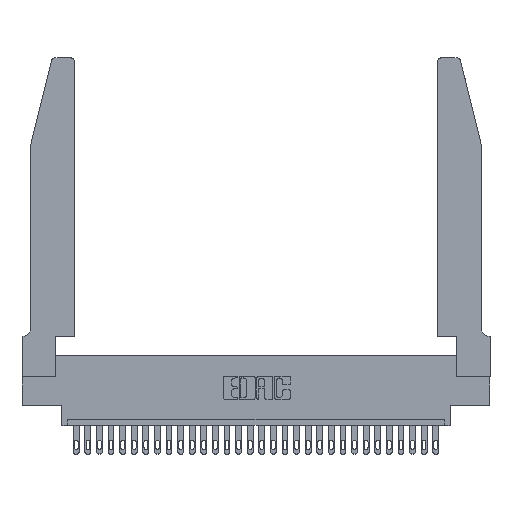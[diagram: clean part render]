
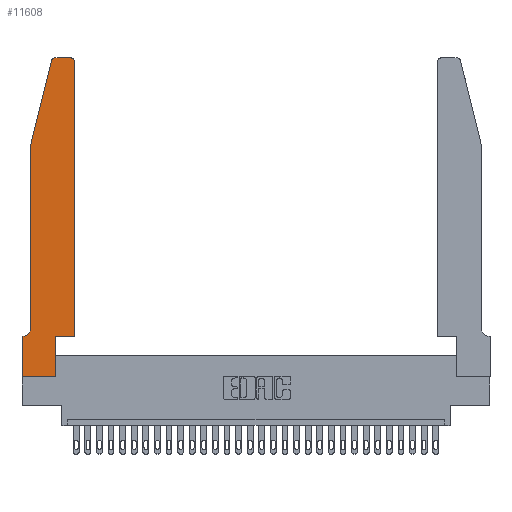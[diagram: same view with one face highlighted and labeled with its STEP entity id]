
A CAD part, top view. The second image highlights one B-rep face of the part: STEP entity #11608.
In plain terms, the highlighted planar face has unit normal (0, 0, 1).
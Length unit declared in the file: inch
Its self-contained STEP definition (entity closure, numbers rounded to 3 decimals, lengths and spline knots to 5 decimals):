
#44 = DIRECTION ( 'NONE',  ( 0., 0., 1. ) ) ;
#209 = EDGE_CURVE ( 'NONE', #25080, #17520, #10941, .T. ) ;
#1206 = VECTOR ( 'NONE', #19951, 39.37008 ) ;
#1261 = DIRECTION ( 'NONE',  ( -0.239, -0.971, 0. ) ) ;
#1425 = DIRECTION ( 'NONE',  ( 0., 1., 0. ) ) ;
#1489 = CARTESIAN_POINT ( 'NONE',  ( 0.2605, 2.75, 0.37 ) ) ;
#1641 = DIRECTION ( 'NONE',  ( 0., 0., 1. ) ) ;
#1795 = VECTOR ( 'NONE', #22745, 39.37008 ) ;
#1859 = VERTEX_POINT ( 'NONE', #10615 ) ;
#1903 = DIRECTION ( 'NONE',  ( -1., 0., 0. ) ) ;
#2166 = CARTESIAN_POINT ( 'NONE',  ( 0.4205, 2.75, 0.37 ) ) ;
#2800 = EDGE_CURVE ( 'NONE', #15365, #28196, #10460, .T. ) ;
#3085 = CARTESIAN_POINT ( 'NONE',  ( 0.4205, 2.72, 0.37 ) ) ;
#3273 = EDGE_CURVE ( 'NONE', #1859, #25080, #15148, .T. ) ;
#3616 = AXIS2_PLACEMENT_3D ( 'NONE', #21990, #12511, #14971 ) ;
#3809 = FACE_OUTER_BOUND ( 'NONE', #16440, .T. ) ;
#3817 = CARTESIAN_POINT ( 'NONE',  ( 0., 0., 0.37 ) ) ;
#4586 = CARTESIAN_POINT ( 'NONE',  ( 0., 0., 0.37 ) ) ;
#4799 = DIRECTION ( 'NONE',  ( 1., 0., 0. ) ) ;
#4923 = ORIENTED_EDGE ( 'NONE', *, *, #209, .T. ) ;
#5251 = EDGE_CURVE ( 'NONE', #9462, #13930, #16127, .T. ) ;
#5314 = DIRECTION ( 'NONE',  ( 0., 0., 1. ) ) ;
#5408 = EDGE_CURVE ( 'NONE', #6255, #11802, #26796, .T. ) ;
#6255 = VERTEX_POINT ( 'NONE', #23559 ) ;
#6917 = CARTESIAN_POINT ( 'NONE',  ( 0.0755, 2., 0.37 ) ) ;
#7028 = ORIENTED_EDGE ( 'NONE', *, *, #5408, .T. ) ;
#7050 = CARTESIAN_POINT ( 'NONE',  ( 0.0755, 0.42, 0.37 ) ) ;
#7767 = EDGE_CURVE ( 'NONE', #28196, #6255, #18661, .T. ) ;
#8279 = EDGE_CURVE ( 'NONE', #29301, #21750, #18254, .T. ) ;
#9185 = VECTOR ( 'NONE', #1425, 39.37008 ) ;
#9462 = VERTEX_POINT ( 'NONE', #4586 ) ;
#9685 = ORIENTED_EDGE ( 'NONE', *, *, #7767, .T. ) ;
#10228 = VECTOR ( 'NONE', #27423, 39.37008 ) ;
#10342 = AXIS2_PLACEMENT_3D ( 'NONE', #3085, #5314, #21494 ) ;
#10460 = LINE ( 'NONE', #24172, #22568 ) ;
#10615 = CARTESIAN_POINT ( 'NONE',  ( 0.4505, 2.72, 0.37 ) ) ;
#10941 = LINE ( 'NONE', #1489, #10228 ) ;
#10971 = CARTESIAN_POINT ( 'NONE',  ( 0.284, 2.72, 0.37 ) ) ;
#11608 = ADVANCED_FACE ( 'NONE', ( #3809 ), #14278, .T. ) ;
#11760 = CIRCLE ( 'NONE', #26680, 0.03 ) ;
#11802 = VERTEX_POINT ( 'NONE', #21668 ) ;
#12511 = DIRECTION ( 'NONE',  ( 0., 0., -1. ) ) ;
#12538 = ORIENTED_EDGE ( 'NONE', *, *, #24192, .T. ) ;
#13164 = DIRECTION ( 'NONE',  ( 0., -1., 0. ) ) ;
#13202 = DIRECTION ( 'NONE',  ( 1., 0., 0. ) ) ;
#13220 = LINE ( 'NONE', #3817, #22057 ) ;
#13282 = CARTESIAN_POINT ( 'NONE',  ( 0.4505, 0.35, 0.37 ) ) ;
#13402 = CARTESIAN_POINT ( 'NONE',  ( 0.4505, 0.35, 0.37 ) ) ;
#13490 = CARTESIAN_POINT ( 'NONE',  ( 0.0755, 0.35, 0.37 ) ) ;
#13930 = VERTEX_POINT ( 'NONE', #18449 ) ;
#14278 = PLANE ( 'NONE',  #28751 ) ;
#14523 = LINE ( 'NONE', #13282, #1795 ) ;
#14741 = ORIENTED_EDGE ( 'NONE', *, *, #8279, .T. ) ;
#14971 = DIRECTION ( 'NONE',  ( -1., 0., 0. ) ) ;
#15065 = ORIENTED_EDGE ( 'NONE', *, *, #20690, .T. ) ;
#15148 = CIRCLE ( 'NONE', #10342, 0.03 ) ;
#15365 = VERTEX_POINT ( 'NONE', #6917 ) ;
#16127 = LINE ( 'NONE', #24570, #1206 ) ;
#16250 = EDGE_CURVE ( 'NONE', #18499, #15365, #19792, .T. ) ;
#16440 = EDGE_LOOP ( 'NONE', ( #4923, #27870, #22645, #22675, #9685, #7028, #12538, #18382, #22742, #14741, #15065, #27743 ) ) ;
#17520 = VERTEX_POINT ( 'NONE', #24271 ) ;
#17816 = DIRECTION ( 'NONE',  ( 1., 0., 0. ) ) ;
#18254 = LINE ( 'NONE', #13402, #20851 ) ;
#18382 = ORIENTED_EDGE ( 'NONE', *, *, #5251, .T. ) ;
#18449 = CARTESIAN_POINT ( 'NONE',  ( 0.2865, 0., 0.37 ) ) ;
#18499 = VERTEX_POINT ( 'NONE', #23398 ) ;
#18661 = CIRCLE ( 'NONE', #3616, 0.07 ) ;
#19641 = DIRECTION ( 'NONE',  ( 0., -1., 0. ) ) ;
#19792 = LINE ( 'NONE', #24638, #28962 ) ;
#19909 = CARTESIAN_POINT ( 'NONE',  ( 0.2865, 0.35, 0.37 ) ) ;
#19951 = DIRECTION ( 'NONE',  ( 1., 0., 0. ) ) ;
#20690 = EDGE_CURVE ( 'NONE', #21750, #1859, #14523, .T. ) ;
#20851 = VECTOR ( 'NONE', #13202, 39.37008 ) ;
#21063 = CARTESIAN_POINT ( 'NONE',  ( 0., 0.35, 0.37 ) ) ;
#21494 = DIRECTION ( 'NONE',  ( 1., 0., 0. ) ) ;
#21668 = CARTESIAN_POINT ( 'NONE',  ( 0., 0.35, 0.37 ) ) ;
#21750 = VERTEX_POINT ( 'NONE', #24810 ) ;
#21990 = CARTESIAN_POINT ( 'NONE',  ( 0.0055, 0.42, 0.37 ) ) ;
#22057 = VECTOR ( 'NONE', #13164, 39.37008 ) ;
#22568 = VECTOR ( 'NONE', #19641, 39.37008 ) ;
#22645 = ORIENTED_EDGE ( 'NONE', *, *, #16250, .T. ) ;
#22675 = ORIENTED_EDGE ( 'NONE', *, *, #2800, .T. ) ;
#22742 = ORIENTED_EDGE ( 'NONE', *, *, #29638, .T. ) ;
#22745 = DIRECTION ( 'NONE',  ( 0., 1., 0. ) ) ;
#23398 = CARTESIAN_POINT ( 'NONE',  ( 0.25487, 2.72718, 0.37 ) ) ;
#23559 = CARTESIAN_POINT ( 'NONE',  ( 0.0055, 0.35, 0.37 ) ) ;
#24172 = CARTESIAN_POINT ( 'NONE',  ( 0.0755, 2., 0.37 ) ) ;
#24192 = EDGE_CURVE ( 'NONE', #11802, #9462, #13220, .T. ) ;
#24271 = CARTESIAN_POINT ( 'NONE',  ( 0.284, 2.75, 0.37 ) ) ;
#24570 = CARTESIAN_POINT ( 'NONE',  ( 0., 0., 0.37 ) ) ;
#24638 = CARTESIAN_POINT ( 'NONE',  ( 0.0755, 2., 0.37 ) ) ;
#24810 = CARTESIAN_POINT ( 'NONE',  ( 0.4505, 0.35, 0.37 ) ) ;
#25080 = VERTEX_POINT ( 'NONE', #2166 ) ;
#26369 = CARTESIAN_POINT ( 'NONE',  ( 0.2865, 0.35, 0.37 ) ) ;
#26680 = AXIS2_PLACEMENT_3D ( 'NONE', #10971, #1641, #17816 ) ;
#26796 = LINE ( 'NONE', #13490, #27518 ) ;
#27423 = DIRECTION ( 'NONE',  ( -1., 0., 0. ) ) ;
#27518 = VECTOR ( 'NONE', #1903, 39.37008 ) ;
#27743 = ORIENTED_EDGE ( 'NONE', *, *, #3273, .T. ) ;
#27870 = ORIENTED_EDGE ( 'NONE', *, *, #28022, .T. ) ;
#28022 = EDGE_CURVE ( 'NONE', #17520, #18499, #11760, .T. ) ;
#28196 = VERTEX_POINT ( 'NONE', #7050 ) ;
#28751 = AXIS2_PLACEMENT_3D ( 'NONE', #21063, #44, #4799 ) ;
#28962 = VECTOR ( 'NONE', #1261, 39.37008 ) ;
#29301 = VERTEX_POINT ( 'NONE', #19909 ) ;
#29625 = LINE ( 'NONE', #26369, #9185 ) ;
#29638 = EDGE_CURVE ( 'NONE', #13930, #29301, #29625, .T. ) ;
